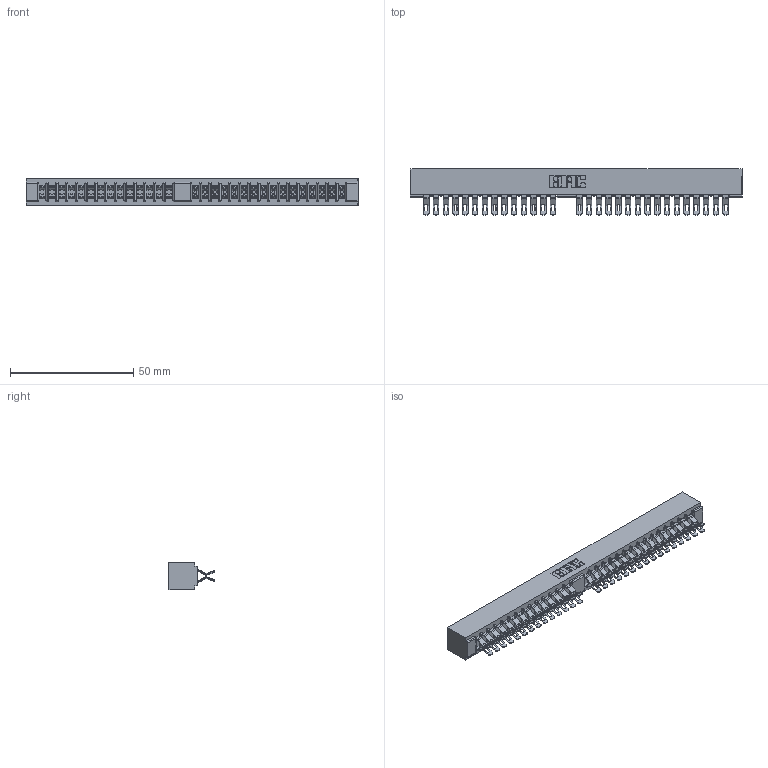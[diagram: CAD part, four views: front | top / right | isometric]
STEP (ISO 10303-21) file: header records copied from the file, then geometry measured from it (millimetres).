
FILE_DESCRIPTION (( 'STEP AP203' ), '1' );
FILE_NAME ('310-060-555-201.STEP', '2020-03-25T14:07:22', ( '' ), ( '' ), 'SwSTEP 2.0', 'SolidWorks 2016', '' );
FILE_SCHEMA (( 'CONFIG_CONTROL_DESIGN' ));
Length unit declared in the file: millimetre
Products named in the file (3): 307-290-001_555; 310-060-555-201; 310 Part_No Mounting Lugs
Assembly tree (61 placements, depth 2):
  310-060-555-201
    310 Part_No Mounting Lugs
    307-290-001_555  x60
Bounding box: 134.92 x 18.69 x 10.97 mm (x, y, z)
Volume: 12189.1 mm3; surface area: 18018.4 mm2
Topology: 61 solids, 61 shells, 3818 faces, 11197 edges, 7294 vertices
Faces by surface type: plane 2120, cylinder 1634, sphere 64
Entity records: 28843 total; most frequent: CARTESIAN_POINT 4727, ORIENTED_EDGE 4684, DIRECTION 4642, EDGE_CURVE 2342, VECTOR 1788, LINE 1788, VERTEX_POINT 1512, AXIS2_PLACEMENT_3D 1427
